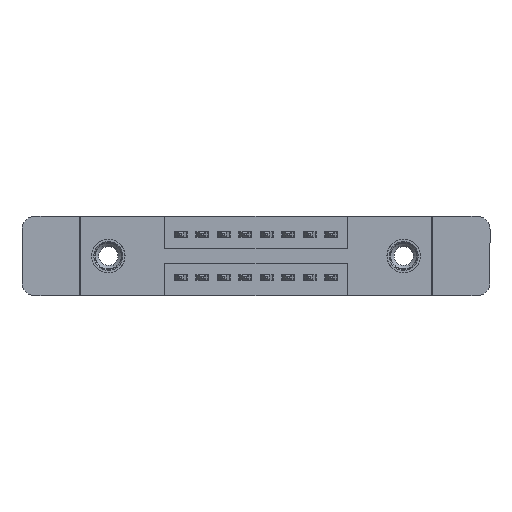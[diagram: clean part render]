
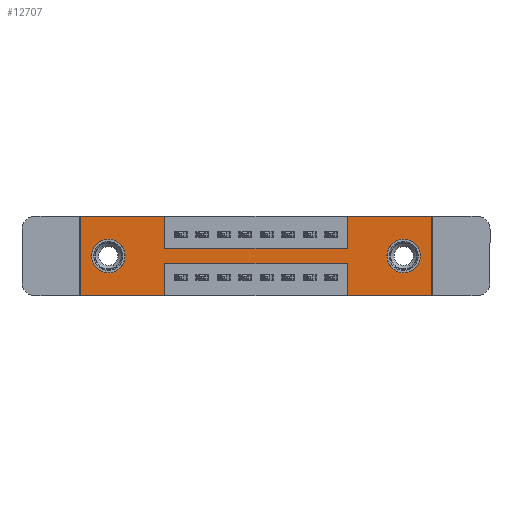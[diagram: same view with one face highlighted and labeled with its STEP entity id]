
A CAD part, front view. The second image highlights one B-rep face of the part: STEP entity #12707.
In plain terms, the highlighted planar face has unit normal (0, -1, 0).
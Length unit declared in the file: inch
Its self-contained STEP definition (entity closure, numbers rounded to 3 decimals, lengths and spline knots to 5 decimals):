
#158 = EDGE_CURVE ( 'NONE', #15288, #13271, #2020, .T. ) ;
#266 = LINE ( 'NONE', #2323, #9731 ) ;
#482 = VECTOR ( 'NONE', #7114, 39.37008 ) ;
#543 = VERTEX_POINT ( 'NONE', #11155 ) ;
#786 = EDGE_CURVE ( 'NONE', #8349, #11618, #11532, .T. ) ;
#939 = CARTESIAN_POINT ( 'NONE',  ( 1.2425, 0., -0.37 ) ) ;
#993 = DIRECTION ( 'NONE',  ( 0., 1., 0. ) ) ;
#1055 = VERTEX_POINT ( 'NONE', #6031 ) ;
#1074 = DIRECTION ( 'NONE',  ( -1., 0., 0. ) ) ;
#1091 = AXIS2_PLACEMENT_3D ( 'NONE', #12728, #5291, #13958 ) ;
#1127 = DIRECTION ( 'NONE',  ( 0., 0., 1. ) ) ;
#1254 = EDGE_CURVE ( 'NONE', #8352, #4755, #6076, .T. ) ;
#1288 = LINE ( 'NONE', #10994, #7893 ) ;
#1599 = LINE ( 'NONE', #6938, #11078 ) ;
#1663 = ORIENTED_EDGE ( 'NONE', *, *, #15118, .F. ) ;
#1672 = EDGE_LOOP ( 'NONE', ( #6564, #6504 ) ) ;
#1702 = CARTESIAN_POINT ( 'NONE',  ( 1.635, 0., -0.37 ) ) ;
#1833 = LINE ( 'NONE', #6131, #4723 ) ;
#2020 = LINE ( 'NONE', #10030, #13882 ) ;
#2023 = CARTESIAN_POINT ( 'NONE',  ( 0.3925, 0., -0.15 ) ) ;
#2097 = CARTESIAN_POINT ( 'NONE',  ( 0., 0., -0.37 ) ) ;
#2278 = VERTEX_POINT ( 'NONE', #3559 ) ;
#2323 = CARTESIAN_POINT ( 'NONE',  ( 0., 0., 0. ) ) ;
#2333 = DIRECTION ( 'NONE',  ( 1., 0., 0. ) ) ;
#2339 = VECTOR ( 'NONE', #2740, 39.37008 ) ;
#2740 = DIRECTION ( 'NONE',  ( -1., 0., 0. ) ) ;
#2741 = CARTESIAN_POINT ( 'NONE',  ( 0.13, 0., -0.107 ) ) ;
#2950 = EDGE_CURVE ( 'NONE', #4961, #15288, #8162, .T. ) ;
#3070 = ORIENTED_EDGE ( 'NONE', *, *, #9262, .F. ) ;
#3276 = AXIS2_PLACEMENT_3D ( 'NONE', #8427, #993, #9655 ) ;
#3370 = DIRECTION ( 'NONE',  ( 0., 1., 0. ) ) ;
#3452 = EDGE_LOOP ( 'NONE', ( #11277, #10884, #14367, #13663, #13841, #1663, #4213, #7472, #8062, #3070, #6950, #11608 ) ) ;
#3559 = CARTESIAN_POINT ( 'NONE',  ( 0., 0., -0.37 ) ) ;
#3587 = VECTOR ( 'NONE', #10707, 39.37008 ) ;
#4189 = CARTESIAN_POINT ( 'NONE',  ( 1.505, 0., -0.107 ) ) ;
#4213 = ORIENTED_EDGE ( 'NONE', *, *, #10226, .F. ) ;
#4230 = FACE_OUTER_BOUND ( 'NONE', #3452, .T. ) ;
#4425 = CARTESIAN_POINT ( 'NONE',  ( 0.3925, 0., 0. ) ) ;
#4617 = FACE_BOUND ( 'NONE', #1672, .T. ) ;
#4723 = VECTOR ( 'NONE', #9863, 39.37008 ) ;
#4755 = VERTEX_POINT ( 'NONE', #7628 ) ;
#4915 = VERTEX_POINT ( 'NONE', #14543 ) ;
#4961 = VERTEX_POINT ( 'NONE', #9659 ) ;
#5291 = DIRECTION ( 'NONE',  ( 0., 1., 0. ) ) ;
#5702 = EDGE_CURVE ( 'NONE', #7771, #13688, #1288, .T. ) ;
#5954 = AXIS2_PLACEMENT_3D ( 'NONE', #10796, #3370, #12053 ) ;
#6031 = CARTESIAN_POINT ( 'NONE',  ( 0., 0., 0. ) ) ;
#6076 = CIRCLE ( 'NONE', #1091, 0.078 ) ;
#6131 = CARTESIAN_POINT ( 'NONE',  ( 1.635, 0., 0. ) ) ;
#6443 = CIRCLE ( 'NONE', #3276, 0.078 ) ;
#6504 = ORIENTED_EDGE ( 'NONE', *, *, #9889, .T. ) ;
#6564 = ORIENTED_EDGE ( 'NONE', *, *, #8648, .T. ) ;
#6773 = EDGE_CURVE ( 'NONE', #13271, #2278, #11568, .T. ) ;
#6815 = DIRECTION ( 'NONE',  ( -1., 0., 0. ) ) ;
#6848 = CIRCLE ( 'NONE', #11157, 0.078 ) ;
#6938 = CARTESIAN_POINT ( 'NONE',  ( 0., 0., 0. ) ) ;
#6946 = CARTESIAN_POINT ( 'NONE',  ( 1.2425, 0., -0.15 ) ) ;
#6950 = ORIENTED_EDGE ( 'NONE', *, *, #8636, .F. ) ;
#7081 = PLANE ( 'NONE',  #14594 ) ;
#7114 = DIRECTION ( 'NONE',  ( 0., 0., 1. ) ) ;
#7276 = EDGE_CURVE ( 'NONE', #12765, #7771, #15238, .T. ) ;
#7453 = LINE ( 'NONE', #939, #482 ) ;
#7472 = ORIENTED_EDGE ( 'NONE', *, *, #5702, .F. ) ;
#7628 = CARTESIAN_POINT ( 'NONE',  ( 1.505, 0., -0.263 ) ) ;
#7771 = VERTEX_POINT ( 'NONE', #2023 ) ;
#7816 = EDGE_CURVE ( 'NONE', #4755, #8352, #14056, .T. ) ;
#7839 = EDGE_CURVE ( 'NONE', #11618, #4961, #7453, .T. ) ;
#7887 = VECTOR ( 'NONE', #1074, 39.37008 ) ;
#7893 = VECTOR ( 'NONE', #2333, 39.37008 ) ;
#7894 = CARTESIAN_POINT ( 'NONE',  ( 0.3925, 0., -0.22 ) ) ;
#8016 = CARTESIAN_POINT ( 'NONE',  ( 0., 0., -0.37 ) ) ;
#8036 = EDGE_CURVE ( 'NONE', #4915, #8349, #1833, .T. ) ;
#8062 = ORIENTED_EDGE ( 'NONE', *, *, #7276, .F. ) ;
#8162 = LINE ( 'NONE', #7894, #2339 ) ;
#8233 = VECTOR ( 'NONE', #6815, 39.37008 ) ;
#8305 = DIRECTION ( 'NONE',  ( 0., 0., 1. ) ) ;
#8329 = DIRECTION ( 'NONE',  ( 0., 0., -1. ) ) ;
#8349 = VERTEX_POINT ( 'NONE', #1702 ) ;
#8352 = VERTEX_POINT ( 'NONE', #4189 ) ;
#8427 = CARTESIAN_POINT ( 'NONE',  ( 0.13, 0., -0.185 ) ) ;
#8439 = CARTESIAN_POINT ( 'NONE',  ( 0.3925, 0., 0. ) ) ;
#8499 = ORIENTED_EDGE ( 'NONE', *, *, #7816, .T. ) ;
#8561 = DIRECTION ( 'NONE',  ( 0., 1., 0. ) ) ;
#8636 = EDGE_CURVE ( 'NONE', #2278, #1055, #266, .T. ) ;
#8648 = EDGE_CURVE ( 'NONE', #13049, #11534, #6848, .T. ) ;
#8806 = DIRECTION ( 'NONE',  ( 0., 0., -1. ) ) ;
#9036 = VECTOR ( 'NONE', #13111, 39.37008 ) ;
#9262 = EDGE_CURVE ( 'NONE', #1055, #12765, #1599, .T. ) ;
#9468 = CARTESIAN_POINT ( 'NONE',  ( 0., 0., 0. ) ) ;
#9655 = DIRECTION ( 'NONE',  ( 0., 0., 1. ) ) ;
#9659 = CARTESIAN_POINT ( 'NONE',  ( 1.2425, 0., -0.22 ) ) ;
#9731 = VECTOR ( 'NONE', #10985, 39.37008 ) ;
#9756 = CARTESIAN_POINT ( 'NONE',  ( 0.13, 0., -0.263 ) ) ;
#9863 = DIRECTION ( 'NONE',  ( 0., 0., -1. ) ) ;
#9883 = CARTESIAN_POINT ( 'NONE',  ( 0.3925, 0., -0.22 ) ) ;
#9889 = EDGE_CURVE ( 'NONE', #11534, #13049, #6443, .T. ) ;
#9924 = CARTESIAN_POINT ( 'NONE',  ( 1.2425, 0., -0.37 ) ) ;
#10030 = CARTESIAN_POINT ( 'NONE',  ( 0.3925, 0., -0.37 ) ) ;
#10185 = LINE ( 'NONE', #9468, #3587 ) ;
#10226 = EDGE_CURVE ( 'NONE', #13688, #543, #11676, .T. ) ;
#10707 = DIRECTION ( 'NONE',  ( 1., 0., 0. ) ) ;
#10796 = CARTESIAN_POINT ( 'NONE',  ( 1.505, 0., -0.185 ) ) ;
#10884 = ORIENTED_EDGE ( 'NONE', *, *, #2950, .F. ) ;
#10985 = DIRECTION ( 'NONE',  ( 0., 0., 1. ) ) ;
#10994 = CARTESIAN_POINT ( 'NONE',  ( 0.3925, 0., -0.15 ) ) ;
#11078 = VECTOR ( 'NONE', #14451, 39.37008 ) ;
#11155 = CARTESIAN_POINT ( 'NONE',  ( 1.2425, 0., 0. ) ) ;
#11157 = AXIS2_PLACEMENT_3D ( 'NONE', #15978, #8561, #1127 ) ;
#11277 = ORIENTED_EDGE ( 'NONE', *, *, #158, .F. ) ;
#11532 = LINE ( 'NONE', #8016, #8233 ) ;
#11534 = VERTEX_POINT ( 'NONE', #9756 ) ;
#11568 = LINE ( 'NONE', #12192, #7887 ) ;
#11608 = ORIENTED_EDGE ( 'NONE', *, *, #6773, .F. ) ;
#11618 = VERTEX_POINT ( 'NONE', #9924 ) ;
#11676 = LINE ( 'NONE', #12005, #14200 ) ;
#11894 = CARTESIAN_POINT ( 'NONE',  ( 0.3925, 0., -0.37 ) ) ;
#12005 = CARTESIAN_POINT ( 'NONE',  ( 1.2425, 0., 0. ) ) ;
#12053 = DIRECTION ( 'NONE',  ( 0., 0., -1. ) ) ;
#12192 = CARTESIAN_POINT ( 'NONE',  ( 0., 0., -0.37 ) ) ;
#12707 = ADVANCED_FACE ( 'NONE', ( #13732, #4617, #4230 ), #7081, .T. ) ;
#12728 = CARTESIAN_POINT ( 'NONE',  ( 1.505, 0., -0.185 ) ) ;
#12765 = VERTEX_POINT ( 'NONE', #8439 ) ;
#13049 = VERTEX_POINT ( 'NONE', #2741 ) ;
#13111 = DIRECTION ( 'NONE',  ( 0., 0., -1. ) ) ;
#13271 = VERTEX_POINT ( 'NONE', #11894 ) ;
#13663 = ORIENTED_EDGE ( 'NONE', *, *, #786, .F. ) ;
#13688 = VERTEX_POINT ( 'NONE', #6946 ) ;
#13732 = FACE_BOUND ( 'NONE', #13876, .T. ) ;
#13841 = ORIENTED_EDGE ( 'NONE', *, *, #8036, .F. ) ;
#13876 = EDGE_LOOP ( 'NONE', ( #14132, #8499 ) ) ;
#13882 = VECTOR ( 'NONE', #8806, 39.37008 ) ;
#13958 = DIRECTION ( 'NONE',  ( 0., 0., -1. ) ) ;
#14056 = CIRCLE ( 'NONE', #5954, 0.078 ) ;
#14132 = ORIENTED_EDGE ( 'NONE', *, *, #1254, .T. ) ;
#14200 = VECTOR ( 'NONE', #8305, 39.37008 ) ;
#14367 = ORIENTED_EDGE ( 'NONE', *, *, #7839, .F. ) ;
#14451 = DIRECTION ( 'NONE',  ( 1., 0., 0. ) ) ;
#14543 = CARTESIAN_POINT ( 'NONE',  ( 1.635, 0., 0. ) ) ;
#14594 = AXIS2_PLACEMENT_3D ( 'NONE', #2097, #15752, #8329 ) ;
#15118 = EDGE_CURVE ( 'NONE', #543, #4915, #10185, .T. ) ;
#15238 = LINE ( 'NONE', #4425, #9036 ) ;
#15288 = VERTEX_POINT ( 'NONE', #9883 ) ;
#15752 = DIRECTION ( 'NONE',  ( 0., -1., 0. ) ) ;
#15978 = CARTESIAN_POINT ( 'NONE',  ( 0.13, 0., -0.185 ) ) ;
